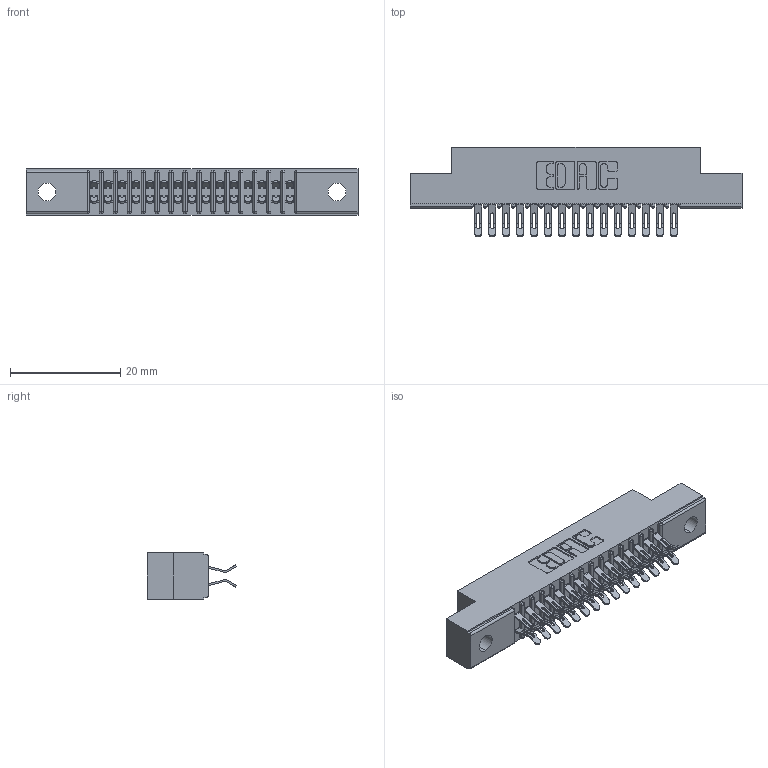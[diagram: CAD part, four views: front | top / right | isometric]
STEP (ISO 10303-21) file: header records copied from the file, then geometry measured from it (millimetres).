
FILE_DESCRIPTION (( 'STEP AP203' ), '1' );
FILE_NAME ('391-030-555-202.STEP', '2018-08-08T21:40:00', ( '' ), ( '' ), 'SwSTEP 2.0', 'SolidWorks 2016', '' );
FILE_SCHEMA (( 'CONFIG_CONTROL_DESIGN' ));
Length unit declared in the file: inch
Products named in the file (3): 341 Part_.128 (3.25) Dia Mounting Holes; 341-292-001_341-292-155; 391-030-555-202
Assembly tree (31 placements, depth 2):
  391-030-555-202
    341 Part_.128 (3.25) Dia Mounting Holes
    341-292-001_341-292-155  x30
Bounding box: 60.33 x 16.31 x 8.38 mm (x, y, z)
Volume: 3451.5 mm3; surface area: 6752.2 mm2
Topology: 31 solids, 31 shells, 2456 faces, 7321 edges, 4766 vertices
Faces by surface type: plane 1328, cylinder 1068, sphere 32, torus 28
Entity records: 22222 total; most frequent: CARTESIAN_POINT 3711, ORIENTED_EDGE 3674, DIRECTION 3611, EDGE_CURVE 1837, LINE 1439, VECTOR 1439, VERTEX_POINT 1170, AXIS2_PLACEMENT_3D 1086
